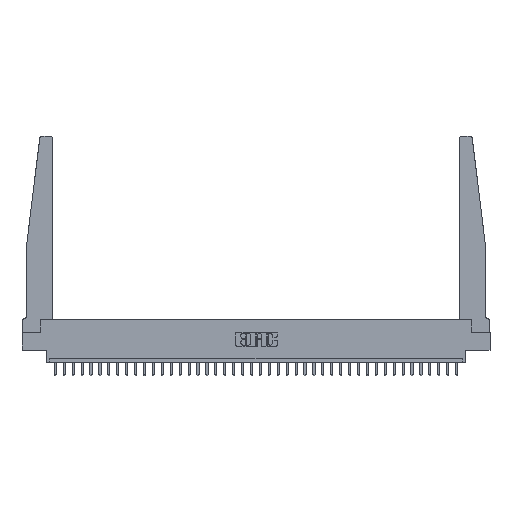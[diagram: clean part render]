
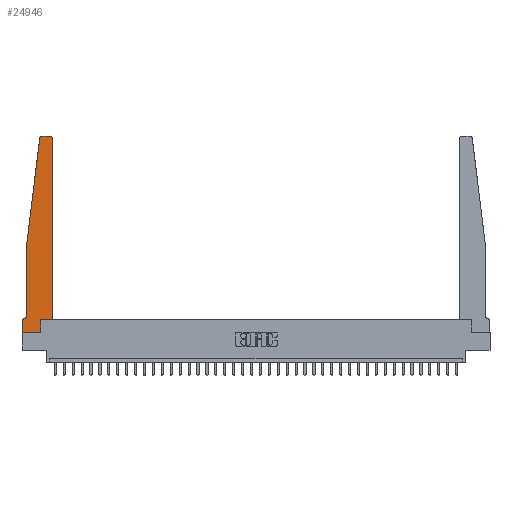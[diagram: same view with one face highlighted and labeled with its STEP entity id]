
A CAD part, top view. The second image highlights one B-rep face of the part: STEP entity #24946.
In plain terms, the highlighted planar face has unit normal (0, 0, 1).
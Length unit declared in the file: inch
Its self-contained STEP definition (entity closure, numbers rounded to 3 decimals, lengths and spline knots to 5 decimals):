
#85 = VECTOR ( 'NONE', #9944, 39.37008 ) ;
#125 = DIRECTION ( 'NONE',  ( 0., 0., -1. ) ) ;
#211 = VERTEX_POINT ( 'NONE', #25742 ) ;
#451 = CARTESIAN_POINT ( 'NONE',  ( 0.065, 1.25, 0.37 ) ) ;
#482 = CARTESIAN_POINT ( 'NONE',  ( 0.27653, 2.75, 0.37 ) ) ;
#682 = CARTESIAN_POINT ( 'NONE',  ( 0.065, 0.2375, 0.37 ) ) ;
#854 = LINE ( 'NONE', #19282, #21558 ) ;
#967 = ORIENTED_EDGE ( 'NONE', *, *, #9736, .T. ) ;
#1252 = PLANE ( 'NONE',  #26289 ) ;
#1500 = ORIENTED_EDGE ( 'NONE', *, *, #4073, .T. ) ;
#1709 = DIRECTION ( 'NONE',  ( -0.122, -0.992, 0. ) ) ;
#1898 = CIRCLE ( 'NONE', #8524, 0.03 ) ;
#2481 = VECTOR ( 'NONE', #1709, 39.37008 ) ;
#3062 = DIRECTION ( 'NONE',  ( 1., 0., 0. ) ) ;
#3577 = CARTESIAN_POINT ( 'NONE',  ( 0.395, 2.75, 0.37 ) ) ;
#4002 = ORIENTED_EDGE ( 'NONE', *, *, #28634, .T. ) ;
#4073 = EDGE_CURVE ( 'NONE', #211, #10678, #17041, .T. ) ;
#4283 = AXIS2_PLACEMENT_3D ( 'NONE', #30508, #125, #25204 ) ;
#4420 = VERTEX_POINT ( 'NONE', #28630 ) ;
#4564 = ORIENTED_EDGE ( 'NONE', *, *, #18021, .T. ) ;
#5232 = VERTEX_POINT ( 'NONE', #682 ) ;
#5515 = CARTESIAN_POINT ( 'NONE',  ( 0.2605, 0., 0.37 ) ) ;
#5844 = CARTESIAN_POINT ( 'NONE',  ( 0.425, 0.18, 0.37 ) ) ;
#5874 = VECTOR ( 'NONE', #28200, 39.37008 ) ;
#6456 = DIRECTION ( 'NONE',  ( 0., 1., 0. ) ) ;
#6481 = CARTESIAN_POINT ( 'NONE',  ( 0.065, 0.1875, 0.37 ) ) ;
#7136 = CARTESIAN_POINT ( 'NONE',  ( 0.015, 0.1875, 0.37 ) ) ;
#7140 = CARTESIAN_POINT ( 'NONE',  ( 0., 0., 0.37 ) ) ;
#8137 = VECTOR ( 'NONE', #17828, 39.37008 ) ;
#8524 = AXIS2_PLACEMENT_3D ( 'NONE', #19314, #16682, #18979 ) ;
#8577 = ORIENTED_EDGE ( 'NONE', *, *, #26565, .T. ) ;
#8839 = CARTESIAN_POINT ( 'NONE',  ( 0.2605, 0.18, 0.37 ) ) ;
#9057 = EDGE_CURVE ( 'NONE', #10678, #16162, #27202, .T. ) ;
#9180 = DIRECTION ( 'NONE',  ( 0., 1., 0. ) ) ;
#9197 = ORIENTED_EDGE ( 'NONE', *, *, #9057, .T. ) ;
#9539 = EDGE_CURVE ( 'NONE', #5232, #18204, #29526, .T. ) ;
#9736 = EDGE_CURVE ( 'NONE', #24992, #5232, #25159, .T. ) ;
#9826 = CARTESIAN_POINT ( 'NONE',  ( 0.425, 0.18, 0.37 ) ) ;
#9944 = DIRECTION ( 'NONE',  ( 1., 0., 0. ) ) ;
#9994 = ORIENTED_EDGE ( 'NONE', *, *, #19364, .T. ) ;
#10021 = VECTOR ( 'NONE', #21900, 39.37008 ) ;
#10618 = CARTESIAN_POINT ( 'NONE',  ( 0.27653, 2.72, 0.37 ) ) ;
#10678 = VERTEX_POINT ( 'NONE', #7140 ) ;
#10733 = CARTESIAN_POINT ( 'NONE',  ( 0.25, 2.75, 0.37 ) ) ;
#11214 = CIRCLE ( 'NONE', #13540, 0.03 ) ;
#12027 = VECTOR ( 'NONE', #23391, 39.37008 ) ;
#13540 = AXIS2_PLACEMENT_3D ( 'NONE', #10618, #15751, #3062 ) ;
#14085 = EDGE_CURVE ( 'NONE', #26912, #21732, #17398, .T. ) ;
#15751 = DIRECTION ( 'NONE',  ( 0., 0., 1. ) ) ;
#16162 = VERTEX_POINT ( 'NONE', #5515 ) ;
#16262 = VECTOR ( 'NONE', #28108, 39.37008 ) ;
#16551 = EDGE_CURVE ( 'NONE', #21732, #18757, #17248, .T. ) ;
#16682 = DIRECTION ( 'NONE',  ( 0., 0., 1. ) ) ;
#16950 = CARTESIAN_POINT ( 'NONE',  ( 0.065, 1.25, 0.37 ) ) ;
#17041 = LINE ( 'NONE', #30201, #16262 ) ;
#17248 = LINE ( 'NONE', #9826, #32405 ) ;
#17398 = LINE ( 'NONE', #5844, #5874 ) ;
#17570 = EDGE_CURVE ( 'NONE', #16162, #26912, #854, .T. ) ;
#17828 = DIRECTION ( 'NONE',  ( -1., 0., 0. ) ) ;
#18021 = EDGE_CURVE ( 'NONE', #18204, #211, #27523, .T. ) ;
#18204 = VERTEX_POINT ( 'NONE', #7136 ) ;
#18757 = VERTEX_POINT ( 'NONE', #27336 ) ;
#18979 = DIRECTION ( 'NONE',  ( 1., 0., 0. ) ) ;
#19282 = CARTESIAN_POINT ( 'NONE',  ( 0.2605, 0.18, 0.37 ) ) ;
#19314 = CARTESIAN_POINT ( 'NONE',  ( 0.395, 2.72, 0.37 ) ) ;
#19364 = EDGE_CURVE ( 'NONE', #4420, #24992, #20399, .T. ) ;
#19452 = ORIENTED_EDGE ( 'NONE', *, *, #9539, .T. ) ;
#20399 = LINE ( 'NONE', #16950, #2481 ) ;
#21544 = CARTESIAN_POINT ( 'NONE',  ( 0.425, 0.18, 0.37 ) ) ;
#21558 = VECTOR ( 'NONE', #6456, 39.37008 ) ;
#21732 = VERTEX_POINT ( 'NONE', #21544 ) ;
#21900 = DIRECTION ( 'NONE',  ( -1., 0., 0. ) ) ;
#21950 = ORIENTED_EDGE ( 'NONE', *, *, #17570, .T. ) ;
#22055 = DIRECTION ( 'NONE',  ( 1., 0., 0. ) ) ;
#22159 = CARTESIAN_POINT ( 'NONE',  ( 0.065, 1.25, 0.37 ) ) ;
#23391 = DIRECTION ( 'NONE',  ( 0., -1., 0. ) ) ;
#24297 = DIRECTION ( 'NONE',  ( 0., 0., 1. ) ) ;
#24633 = CARTESIAN_POINT ( 'NONE',  ( 0., 0.1875, 0.37 ) ) ;
#24712 = ORIENTED_EDGE ( 'NONE', *, *, #30519, .T. ) ;
#24946 = ADVANCED_FACE ( 'NONE', ( #30328 ), #1252, .T. ) ;
#24992 = VERTEX_POINT ( 'NONE', #22159 ) ;
#25159 = LINE ( 'NONE', #451, #12027 ) ;
#25204 = DIRECTION ( 'NONE',  ( -1., 0., 0. ) ) ;
#25293 = ORIENTED_EDGE ( 'NONE', *, *, #16551, .T. ) ;
#25742 = CARTESIAN_POINT ( 'NONE',  ( 0., 0.1875, 0.37 ) ) ;
#26289 = AXIS2_PLACEMENT_3D ( 'NONE', #24633, #24297, #22055 ) ;
#26504 = EDGE_LOOP ( 'NONE', ( #4002, #24712, #9994, #967, #19452, #4564, #1500, #9197, #21950, #27521, #25293, #8577 ) ) ;
#26565 = EDGE_CURVE ( 'NONE', #18757, #29265, #1898, .T. ) ;
#26912 = VERTEX_POINT ( 'NONE', #8839 ) ;
#27202 = LINE ( 'NONE', #32421, #85 ) ;
#27336 = CARTESIAN_POINT ( 'NONE',  ( 0.425, 2.72, 0.37 ) ) ;
#27521 = ORIENTED_EDGE ( 'NONE', *, *, #14085, .T. ) ;
#27523 = LINE ( 'NONE', #6481, #10021 ) ;
#28108 = DIRECTION ( 'NONE',  ( 0., -1., 0. ) ) ;
#28200 = DIRECTION ( 'NONE',  ( 1., 0., 0. ) ) ;
#28630 = CARTESIAN_POINT ( 'NONE',  ( 0.24675, 2.72367, 0.37 ) ) ;
#28634 = EDGE_CURVE ( 'NONE', #29265, #31869, #28840, .T. ) ;
#28840 = LINE ( 'NONE', #10733, #8137 ) ;
#29265 = VERTEX_POINT ( 'NONE', #3577 ) ;
#29526 = CIRCLE ( 'NONE', #4283, 0.05 ) ;
#30201 = CARTESIAN_POINT ( 'NONE',  ( 0., 0., 0.37 ) ) ;
#30328 = FACE_OUTER_BOUND ( 'NONE', #26504, .T. ) ;
#30508 = CARTESIAN_POINT ( 'NONE',  ( 0.015, 0.2375, 0.37 ) ) ;
#30519 = EDGE_CURVE ( 'NONE', #31869, #4420, #11214, .T. ) ;
#31869 = VERTEX_POINT ( 'NONE', #482 ) ;
#32405 = VECTOR ( 'NONE', #9180, 39.37008 ) ;
#32421 = CARTESIAN_POINT ( 'NONE',  ( 0., 0., 0.37 ) ) ;
